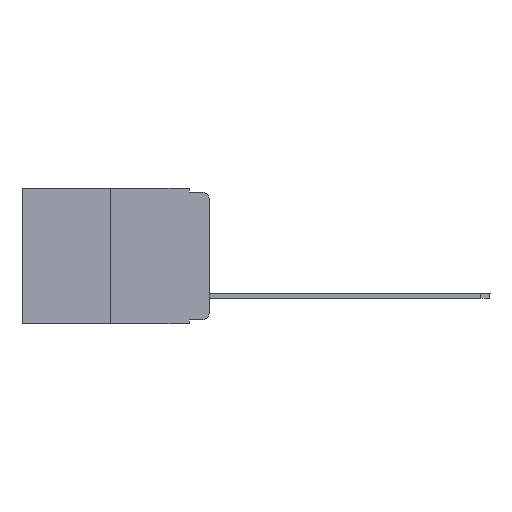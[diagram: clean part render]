
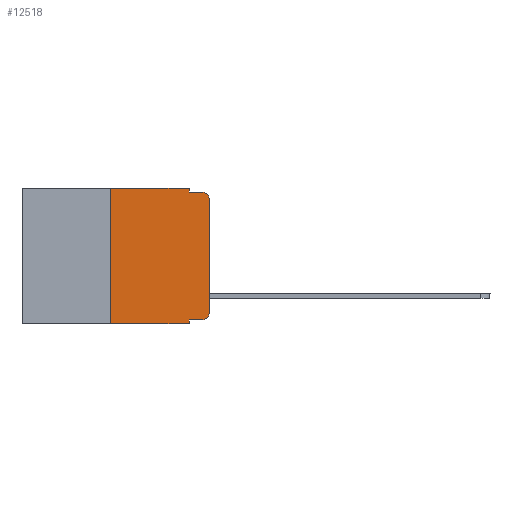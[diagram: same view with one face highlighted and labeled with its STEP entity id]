
A CAD part, left-side view. The second image highlights one B-rep face of the part: STEP entity #12518.
In plain terms, the highlighted planar face has unit normal (-1, 0, 0).
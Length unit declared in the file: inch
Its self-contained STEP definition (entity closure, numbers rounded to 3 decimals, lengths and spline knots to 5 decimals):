
#47 = CARTESIAN_POINT ( 'NONE',  ( 0., 0.051, -0.01 ) ) ;
#427 = CARTESIAN_POINT ( 'NONE',  ( 0., 0.02, -0.01 ) ) ;
#555 = LINE ( 'NONE', #685, #14786 ) ;
#685 = CARTESIAN_POINT ( 'NONE',  ( 0., 0.051, 0. ) ) ;
#744 = ORIENTED_EDGE ( 'NONE', *, *, #5510, .T. ) ;
#1117 = EDGE_LOOP ( 'NONE', ( #744, #5024, #11136, #19880, #23053, #20240, #15028, #15132, #14314, #24380 ) ) ;
#1248 = CIRCLE ( 'NONE', #2047, 0.02 ) ;
#2047 = AXIS2_PLACEMENT_3D ( 'NONE', #14369, #20600, #10984 ) ;
#2141 = VERTEX_POINT ( 'NONE', #14157 ) ;
#2527 = PLANE ( 'NONE',  #2966 ) ;
#2537 = CARTESIAN_POINT ( 'NONE',  ( 0., 0.25, -0.343 ) ) ;
#2608 = EDGE_CURVE ( 'NONE', #24070, #7541, #1248, .T. ) ;
#2645 = CARTESIAN_POINT ( 'NONE',  ( 0., 0., 0. ) ) ;
#2789 = EDGE_CURVE ( 'NONE', #5644, #15231, #8210, .T. ) ;
#2966 = AXIS2_PLACEMENT_3D ( 'NONE', #12493, #21616, #20114 ) ;
#3106 = CARTESIAN_POINT ( 'NONE',  ( 0., 0.25, 0. ) ) ;
#3968 = CARTESIAN_POINT ( 'NONE',  ( 0., 0.051, 0. ) ) ;
#4094 = DIRECTION ( 'NONE',  ( 0., 0., -1. ) ) ;
#4281 = LINE ( 'NONE', #11893, #12140 ) ;
#4749 = AXIS2_PLACEMENT_3D ( 'NONE', #21850, #12121, #14241 ) ;
#5024 = ORIENTED_EDGE ( 'NONE', *, *, #20135, .T. ) ;
#5478 = CARTESIAN_POINT ( 'NONE',  ( 0., 0.051, 0. ) ) ;
#5510 = EDGE_CURVE ( 'NONE', #7541, #13261, #17745, .T. ) ;
#5644 = VERTEX_POINT ( 'NONE', #5478 ) ;
#7343 = VERTEX_POINT ( 'NONE', #18574 ) ;
#7541 = VERTEX_POINT ( 'NONE', #17440 ) ;
#7631 = VECTOR ( 'NONE', #4094, 39.37008 ) ;
#7766 = CARTESIAN_POINT ( 'NONE',  ( 0., 0.051, -0.343 ) ) ;
#8012 = LINE ( 'NONE', #23352, #22079 ) ;
#8210 = LINE ( 'NONE', #3968, #7631 ) ;
#8387 = DIRECTION ( 'NONE',  ( 0., 0., 1. ) ) ;
#8662 = EDGE_CURVE ( 'NONE', #15448, #12345, #19165, .T. ) ;
#9206 = EDGE_CURVE ( 'NONE', #7343, #5644, #4281, .T. ) ;
#10063 = CARTESIAN_POINT ( 'NONE',  ( 0., 0., -0.03 ) ) ;
#10338 = EDGE_CURVE ( 'NONE', #2141, #12345, #555, .T. ) ;
#10350 = VERTEX_POINT ( 'NONE', #427 ) ;
#10702 = DIRECTION ( 'NONE',  ( 0., 0., 1. ) ) ;
#10826 = LINE ( 'NONE', #3106, #19739 ) ;
#10984 = DIRECTION ( 'NONE',  ( 0., 0., -1. ) ) ;
#11117 = VECTOR ( 'NONE', #11753, 39.37008 ) ;
#11136 = ORIENTED_EDGE ( 'NONE', *, *, #11968, .F. ) ;
#11674 = CARTESIAN_POINT ( 'NONE',  ( 0., 0.473, -0.343 ) ) ;
#11753 = DIRECTION ( 'NONE',  ( 0., -1., 0. ) ) ;
#11893 = CARTESIAN_POINT ( 'NONE',  ( 0., 0.473, 0. ) ) ;
#11968 = EDGE_CURVE ( 'NONE', #15231, #10350, #8012, .T. ) ;
#12121 = DIRECTION ( 'NONE',  ( -1., 0., 0. ) ) ;
#12140 = VECTOR ( 'NONE', #19517, 39.37008 ) ;
#12345 = VERTEX_POINT ( 'NONE', #7766 ) ;
#12493 = CARTESIAN_POINT ( 'NONE',  ( 0., 0.473, 0. ) ) ;
#12518 = ADVANCED_FACE ( 'NONE', ( #21982 ), #2527, .F. ) ;
#13009 = EDGE_CURVE ( 'NONE', #15448, #7343, #10826, .T. ) ;
#13261 = VERTEX_POINT ( 'NONE', #10063 ) ;
#13765 = DIRECTION ( 'NONE',  ( 0., 0., -1. ) ) ;
#14157 = CARTESIAN_POINT ( 'NONE',  ( 0., 0.051, -0.333 ) ) ;
#14241 = DIRECTION ( 'NONE',  ( 0., 0., -1. ) ) ;
#14314 = ORIENTED_EDGE ( 'NONE', *, *, #18793, .T. ) ;
#14369 = CARTESIAN_POINT ( 'NONE',  ( 0., 0.02, -0.313 ) ) ;
#14786 = VECTOR ( 'NONE', #13765, 39.37008 ) ;
#15028 = ORIENTED_EDGE ( 'NONE', *, *, #8662, .T. ) ;
#15037 = DIRECTION ( 'NONE',  ( 0., -1., 0. ) ) ;
#15132 = ORIENTED_EDGE ( 'NONE', *, *, #10338, .F. ) ;
#15182 = VECTOR ( 'NONE', #8387, 39.37008 ) ;
#15231 = VERTEX_POINT ( 'NONE', #47 ) ;
#15448 = VERTEX_POINT ( 'NONE', #2537 ) ;
#15990 = DIRECTION ( 'NONE',  ( 0., -1., 0. ) ) ;
#17440 = CARTESIAN_POINT ( 'NONE',  ( 0., 0., -0.313 ) ) ;
#17745 = LINE ( 'NONE', #2645, #15182 ) ;
#18574 = CARTESIAN_POINT ( 'NONE',  ( 0., 0.25, 0. ) ) ;
#18585 = VECTOR ( 'NONE', #15037, 39.37008 ) ;
#18793 = EDGE_CURVE ( 'NONE', #2141, #24070, #21237, .T. ) ;
#19165 = LINE ( 'NONE', #11674, #18585 ) ;
#19498 = CARTESIAN_POINT ( 'NONE',  ( 0., 0.051, -0.333 ) ) ;
#19517 = DIRECTION ( 'NONE',  ( 0., -1., 0. ) ) ;
#19739 = VECTOR ( 'NONE', #10702, 39.37008 ) ;
#19880 = ORIENTED_EDGE ( 'NONE', *, *, #2789, .F. ) ;
#19959 = CIRCLE ( 'NONE', #4749, 0.02 ) ;
#20114 = DIRECTION ( 'NONE',  ( 0., 0., -1. ) ) ;
#20135 = EDGE_CURVE ( 'NONE', #13261, #10350, #19959, .T. ) ;
#20240 = ORIENTED_EDGE ( 'NONE', *, *, #13009, .F. ) ;
#20600 = DIRECTION ( 'NONE',  ( -1., 0., 0. ) ) ;
#21141 = CARTESIAN_POINT ( 'NONE',  ( 0., 0.02, -0.333 ) ) ;
#21237 = LINE ( 'NONE', #19498, #11117 ) ;
#21616 = DIRECTION ( 'NONE',  ( 1., 0., 0. ) ) ;
#21850 = CARTESIAN_POINT ( 'NONE',  ( 0., 0.02, -0.03 ) ) ;
#21982 = FACE_OUTER_BOUND ( 'NONE', #1117, .T. ) ;
#22079 = VECTOR ( 'NONE', #15990, 39.37008 ) ;
#23053 = ORIENTED_EDGE ( 'NONE', *, *, #9206, .F. ) ;
#23352 = CARTESIAN_POINT ( 'NONE',  ( 0., 0.051, -0.01 ) ) ;
#24070 = VERTEX_POINT ( 'NONE', #21141 ) ;
#24380 = ORIENTED_EDGE ( 'NONE', *, *, #2608, .T. ) ;
